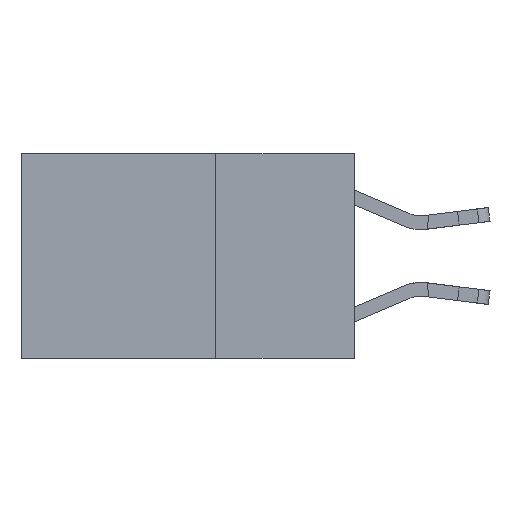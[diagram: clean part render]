
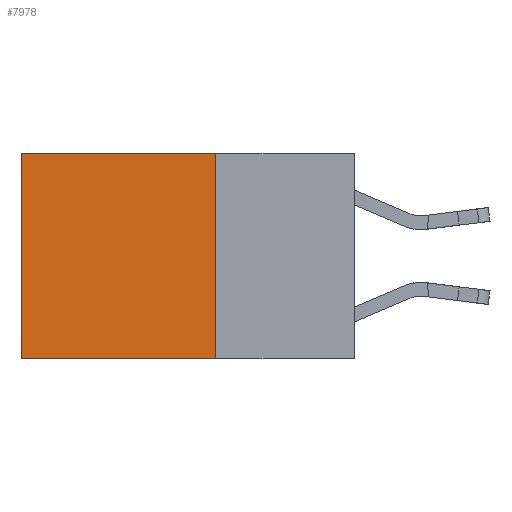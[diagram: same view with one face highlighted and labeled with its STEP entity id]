
A CAD part, left-side view. The second image highlights one B-rep face of the part: STEP entity #7978.
In plain terms, the highlighted planar face has unit normal (-1, 0, 0).
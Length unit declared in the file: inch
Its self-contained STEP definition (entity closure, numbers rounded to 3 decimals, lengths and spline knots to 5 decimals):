
#295 = VERTEX_POINT ( 'NONE', #3464 ) ;
#1428 = PLANE ( 'NONE',  #23141 ) ;
#2394 = LINE ( 'NONE', #13583, #20372 ) ;
#3464 = CARTESIAN_POINT ( 'NONE',  ( 0.2625, 0.6, 0. ) ) ;
#4976 = FACE_OUTER_BOUND ( 'NONE', #5203, .T. ) ;
#4996 = EDGE_CURVE ( 'NONE', #14109, #15519, #9756, .T. ) ;
#5102 = ORIENTED_EDGE ( 'NONE', *, *, #4996, .F. ) ;
#5203 = EDGE_LOOP ( 'NONE', ( #12284, #14017, #5102, #15266 ) ) ;
#5541 = VECTOR ( 'NONE', #14750, 39.37008 ) ;
#5611 = VECTOR ( 'NONE', #7228, 39.37008 ) ;
#5942 = CARTESIAN_POINT ( 'NONE',  ( 0.2625, 0.25, 0. ) ) ;
#6702 = CARTESIAN_POINT ( 'NONE',  ( 0.2625, 0.25, -0.37 ) ) ;
#6936 = CARTESIAN_POINT ( 'NONE',  ( 0.2625, 0.25, 0. ) ) ;
#7097 = LINE ( 'NONE', #16414, #5611 ) ;
#7228 = DIRECTION ( 'NONE',  ( 0., 1., 0. ) ) ;
#7978 = ADVANCED_FACE ( 'NONE', ( #4976 ), #1428, .F. ) ;
#8178 = EDGE_CURVE ( 'NONE', #14109, #295, #2394, .T. ) ;
#8245 = DIRECTION ( 'NONE',  ( 0., 1., 0. ) ) ;
#9123 = VERTEX_POINT ( 'NONE', #11612 ) ;
#9205 = LINE ( 'NONE', #16571, #5541 ) ;
#9756 = LINE ( 'NONE', #18994, #11801 ) ;
#11612 = CARTESIAN_POINT ( 'NONE',  ( 0.2625, 0.6, -0.37 ) ) ;
#11801 = VECTOR ( 'NONE', #13046, 39.37008 ) ;
#12284 = ORIENTED_EDGE ( 'NONE', *, *, #14540, .T. ) ;
#13046 = DIRECTION ( 'NONE',  ( 0., 0., -1. ) ) ;
#13583 = CARTESIAN_POINT ( 'NONE',  ( 0.2625, 0.25, 0. ) ) ;
#14017 = ORIENTED_EDGE ( 'NONE', *, *, #18460, .F. ) ;
#14109 = VERTEX_POINT ( 'NONE', #5942 ) ;
#14540 = EDGE_CURVE ( 'NONE', #295, #9123, #9205, .T. ) ;
#14750 = DIRECTION ( 'NONE',  ( 0., 0., -1. ) ) ;
#15266 = ORIENTED_EDGE ( 'NONE', *, *, #8178, .T. ) ;
#15519 = VERTEX_POINT ( 'NONE', #6702 ) ;
#16414 = CARTESIAN_POINT ( 'NONE',  ( 0.2625, 0.25, -0.37 ) ) ;
#16571 = CARTESIAN_POINT ( 'NONE',  ( 0.2625, 0.6, 0. ) ) ;
#18460 = EDGE_CURVE ( 'NONE', #15519, #9123, #7097, .T. ) ;
#18994 = CARTESIAN_POINT ( 'NONE',  ( 0.2625, 0.25, 0. ) ) ;
#20372 = VECTOR ( 'NONE', #8245, 39.37008 ) ;
#21523 = DIRECTION ( 'NONE',  ( 0., 0., -1. ) ) ;
#23141 = AXIS2_PLACEMENT_3D ( 'NONE', #6936, #23477, #21523 ) ;
#23477 = DIRECTION ( 'NONE',  ( 1., 0., 0. ) ) ;
